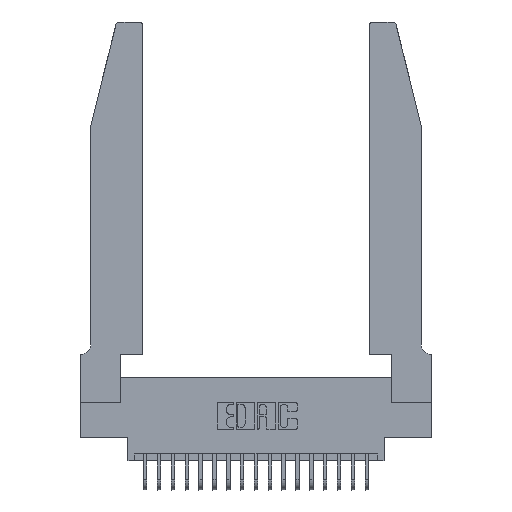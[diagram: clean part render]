
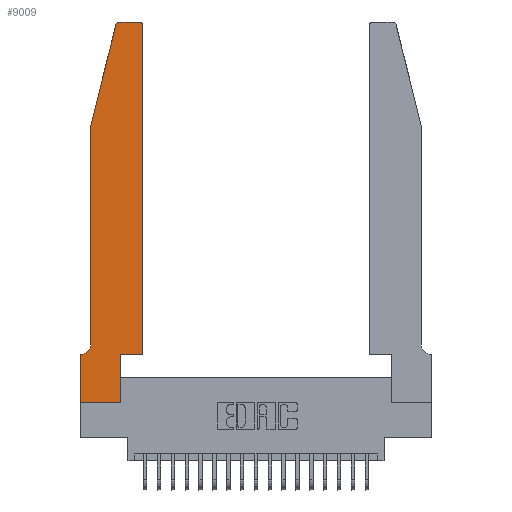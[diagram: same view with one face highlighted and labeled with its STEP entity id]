
A CAD part, top view. The second image highlights one B-rep face of the part: STEP entity #9009.
In plain terms, the highlighted planar face has unit normal (0, 0, 1).
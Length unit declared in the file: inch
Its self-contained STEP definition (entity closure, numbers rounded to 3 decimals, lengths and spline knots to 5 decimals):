
#160 = ORIENTED_EDGE ( 'NONE', *, *, #13060, .T. ) ;
#397 = AXIS2_PLACEMENT_3D ( 'NONE', #20617, #13582, #17223 ) ;
#564 = CIRCLE ( 'NONE', #14909, 0.07 ) ;
#600 = VECTOR ( 'NONE', #5793, 39.37008 ) ;
#620 = CARTESIAN_POINT ( 'NONE',  ( 0.2605, 2.75, 0.37 ) ) ;
#875 = CARTESIAN_POINT ( 'NONE',  ( 0.0055, 0.35, 0.37 ) ) ;
#956 = CARTESIAN_POINT ( 'NONE',  ( 0., 0., 0.37 ) ) ;
#1237 = ORIENTED_EDGE ( 'NONE', *, *, #2668, .T. ) ;
#1504 = VECTOR ( 'NONE', #6275, 39.37008 ) ;
#1607 = VERTEX_POINT ( 'NONE', #19236 ) ;
#2011 = EDGE_CURVE ( 'NONE', #2825, #2198, #23094, .T. ) ;
#2198 = VERTEX_POINT ( 'NONE', #16558 ) ;
#2663 = AXIS2_PLACEMENT_3D ( 'NONE', #6096, #7960, #13389 ) ;
#2668 = EDGE_CURVE ( 'NONE', #12589, #1607, #4531, .T. ) ;
#2825 = VERTEX_POINT ( 'NONE', #16636 ) ;
#2863 = PLANE ( 'NONE',  #10451 ) ;
#3037 = EDGE_LOOP ( 'NONE', ( #13547, #15567, #13107, #160, #12550, #17562, #4196, #3457, #18416, #10556, #1237, #21742 ) ) ;
#3457 = ORIENTED_EDGE ( 'NONE', *, *, #16799, .T. ) ;
#3503 = VERTEX_POINT ( 'NONE', #19094 ) ;
#3971 = EDGE_CURVE ( 'NONE', #3503, #19031, #6082, .T. ) ;
#4037 = DIRECTION ( 'NONE',  ( -1., 0., 0. ) ) ;
#4196 = ORIENTED_EDGE ( 'NONE', *, *, #16034, .T. ) ;
#4255 = EDGE_CURVE ( 'NONE', #6024, #12589, #17334, .T. ) ;
#4350 = CARTESIAN_POINT ( 'NONE',  ( 0.284, 2.75, 0.37 ) ) ;
#4531 = LINE ( 'NONE', #7287, #600 ) ;
#4580 = CARTESIAN_POINT ( 'NONE',  ( 0., 0.35, 0.37 ) ) ;
#4976 = VERTEX_POINT ( 'NONE', #875 ) ;
#5145 = LINE ( 'NONE', #9752, #1504 ) ;
#5179 = DIRECTION ( 'NONE',  ( 1., 0., 0. ) ) ;
#5231 = VECTOR ( 'NONE', #5179, 39.37008 ) ;
#5380 = CARTESIAN_POINT ( 'NONE',  ( 0., 0., 0.37 ) ) ;
#5793 = DIRECTION ( 'NONE',  ( 0., 1., 0. ) ) ;
#5809 = CARTESIAN_POINT ( 'NONE',  ( 0.0755, 0.42, 0.37 ) ) ;
#5859 = CIRCLE ( 'NONE', #397, 0.03 ) ;
#5945 = VECTOR ( 'NONE', #21303, 39.37008 ) ;
#6024 = VERTEX_POINT ( 'NONE', #11209 ) ;
#6082 = LINE ( 'NONE', #620, #8330 ) ;
#6096 = CARTESIAN_POINT ( 'NONE',  ( 0.4205, 2.72, 0.37 ) ) ;
#6275 = DIRECTION ( 'NONE',  ( 0., 1., 0. ) ) ;
#6736 = EDGE_CURVE ( 'NONE', #11732, #6024, #5145, .T. ) ;
#7148 = VECTOR ( 'NONE', #23135, 39.37008 ) ;
#7287 = CARTESIAN_POINT ( 'NONE',  ( 0.4505, 0.35, 0.37 ) ) ;
#7416 = LINE ( 'NONE', #5380, #7148 ) ;
#7780 = CARTESIAN_POINT ( 'NONE',  ( 0.0055, 0.42, 0.37 ) ) ;
#7788 = CARTESIAN_POINT ( 'NONE',  ( 0.0755, 2., 0.37 ) ) ;
#7960 = DIRECTION ( 'NONE',  ( 0., 0., 1. ) ) ;
#8330 = VECTOR ( 'NONE', #14946, 39.37008 ) ;
#8684 = VECTOR ( 'NONE', #13051, 39.37008 ) ;
#8742 = VECTOR ( 'NONE', #12954, 39.37008 ) ;
#9009 = ADVANCED_FACE ( 'NONE', ( #12641 ), #2863, .T. ) ;
#9186 = CARTESIAN_POINT ( 'NONE',  ( 0., 0.35, 0.37 ) ) ;
#9516 = DIRECTION ( 'NONE',  ( 0., 0., -1. ) ) ;
#9669 = EDGE_CURVE ( 'NONE', #19031, #2825, #5859, .T. ) ;
#9752 = CARTESIAN_POINT ( 'NONE',  ( 0.2865, 0.35, 0.37 ) ) ;
#9754 = DIRECTION ( 'NONE',  ( 0., 0., 1. ) ) ;
#10363 = CARTESIAN_POINT ( 'NONE',  ( 0.0755, 2., 0.37 ) ) ;
#10451 = AXIS2_PLACEMENT_3D ( 'NONE', #4580, #9754, #22333 ) ;
#10556 = ORIENTED_EDGE ( 'NONE', *, *, #4255, .T. ) ;
#11176 = LINE ( 'NONE', #19587, #22745 ) ;
#11209 = CARTESIAN_POINT ( 'NONE',  ( 0.2865, 0.35, 0.37 ) ) ;
#11732 = VERTEX_POINT ( 'NONE', #17458 ) ;
#12150 = EDGE_CURVE ( 'NONE', #1607, #3503, #19450, .T. ) ;
#12550 = ORIENTED_EDGE ( 'NONE', *, *, #18864, .T. ) ;
#12589 = VERTEX_POINT ( 'NONE', #16571 ) ;
#12594 = VERTEX_POINT ( 'NONE', #9186 ) ;
#12641 = FACE_OUTER_BOUND ( 'NONE', #3037, .T. ) ;
#12804 = CARTESIAN_POINT ( 'NONE',  ( 0., 0., 0.37 ) ) ;
#12954 = DIRECTION ( 'NONE',  ( 1., 0., 0. ) ) ;
#13051 = DIRECTION ( 'NONE',  ( 0., -1., 0. ) ) ;
#13060 = EDGE_CURVE ( 'NONE', #2198, #16800, #16304, .T. ) ;
#13107 = ORIENTED_EDGE ( 'NONE', *, *, #2011, .T. ) ;
#13389 = DIRECTION ( 'NONE',  ( 1., 0., 0. ) ) ;
#13547 = ORIENTED_EDGE ( 'NONE', *, *, #3971, .T. ) ;
#13582 = DIRECTION ( 'NONE',  ( 0., 0., 1. ) ) ;
#13867 = VERTEX_POINT ( 'NONE', #956 ) ;
#14064 = DIRECTION ( 'NONE',  ( -1., 0., 0. ) ) ;
#14909 = AXIS2_PLACEMENT_3D ( 'NONE', #7780, #9516, #4037 ) ;
#14946 = DIRECTION ( 'NONE',  ( -1., 0., 0. ) ) ;
#15567 = ORIENTED_EDGE ( 'NONE', *, *, #9669, .T. ) ;
#16034 = EDGE_CURVE ( 'NONE', #12594, #13867, #7416, .T. ) ;
#16304 = LINE ( 'NONE', #7788, #8684 ) ;
#16558 = CARTESIAN_POINT ( 'NONE',  ( 0.0755, 2., 0.37 ) ) ;
#16571 = CARTESIAN_POINT ( 'NONE',  ( 0.4505, 0.35, 0.37 ) ) ;
#16636 = CARTESIAN_POINT ( 'NONE',  ( 0.25487, 2.72718, 0.37 ) ) ;
#16799 = EDGE_CURVE ( 'NONE', #13867, #11732, #17776, .T. ) ;
#16800 = VERTEX_POINT ( 'NONE', #5809 ) ;
#17223 = DIRECTION ( 'NONE',  ( 1., 0., 0. ) ) ;
#17334 = LINE ( 'NONE', #19488, #5231 ) ;
#17458 = CARTESIAN_POINT ( 'NONE',  ( 0.2865, 0., 0.37 ) ) ;
#17562 = ORIENTED_EDGE ( 'NONE', *, *, #19322, .T. ) ;
#17776 = LINE ( 'NONE', #12804, #8742 ) ;
#18416 = ORIENTED_EDGE ( 'NONE', *, *, #6736, .T. ) ;
#18864 = EDGE_CURVE ( 'NONE', #16800, #4976, #564, .T. ) ;
#19031 = VERTEX_POINT ( 'NONE', #4350 ) ;
#19094 = CARTESIAN_POINT ( 'NONE',  ( 0.4205, 2.75, 0.37 ) ) ;
#19236 = CARTESIAN_POINT ( 'NONE',  ( 0.4505, 2.72, 0.37 ) ) ;
#19322 = EDGE_CURVE ( 'NONE', #4976, #12594, #11176, .T. ) ;
#19450 = CIRCLE ( 'NONE', #2663, 0.03 ) ;
#19488 = CARTESIAN_POINT ( 'NONE',  ( 0.4505, 0.35, 0.37 ) ) ;
#19587 = CARTESIAN_POINT ( 'NONE',  ( 0.0755, 0.35, 0.37 ) ) ;
#20617 = CARTESIAN_POINT ( 'NONE',  ( 0.284, 2.72, 0.37 ) ) ;
#21303 = DIRECTION ( 'NONE',  ( -0.239, -0.971, 0. ) ) ;
#21742 = ORIENTED_EDGE ( 'NONE', *, *, #12150, .T. ) ;
#22333 = DIRECTION ( 'NONE',  ( 1., 0., 0. ) ) ;
#22745 = VECTOR ( 'NONE', #14064, 39.37008 ) ;
#23094 = LINE ( 'NONE', #10363, #5945 ) ;
#23135 = DIRECTION ( 'NONE',  ( 0., -1., 0. ) ) ;
